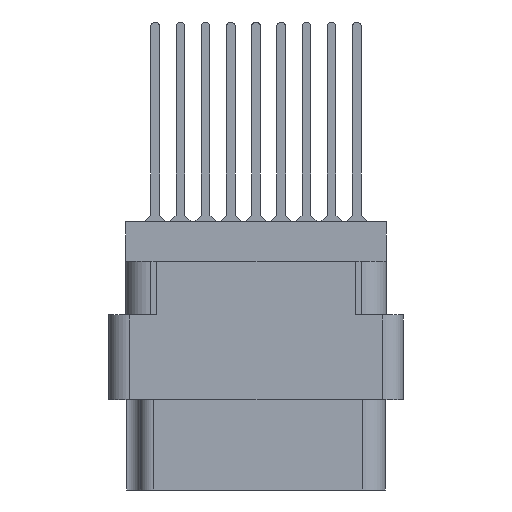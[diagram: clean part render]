
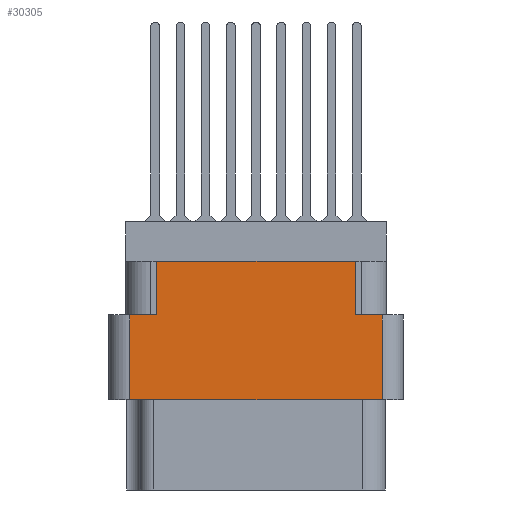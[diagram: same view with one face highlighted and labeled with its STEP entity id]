
A CAD part, left-side view. The second image highlights one B-rep face of the part: STEP entity #30305.
In plain terms, the highlighted planar face has unit normal (-1, 0, 0).
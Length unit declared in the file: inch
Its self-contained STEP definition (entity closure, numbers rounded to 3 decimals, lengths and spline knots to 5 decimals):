
#547 = CARTESIAN_POINT ( 'NONE',  ( -1.296, -0.296, -0.117 ) ) ;
#1099 = CARTESIAN_POINT ( 'NONE',  ( -1.296, -0.438, -0.798 ) ) ;
#1551 = LINE ( 'NONE', #26097, #23637 ) ;
#1974 = DIRECTION ( 'NONE',  ( 0., -1., 0. ) ) ;
#1977 = VECTOR ( 'NONE', #12598, 39.37008 ) ;
#2829 = FACE_OUTER_BOUND ( 'NONE', #41896, .T. ) ;
#2969 = EDGE_CURVE ( 'NONE', #28040, #22588, #7296, .T. ) ;
#3328 = CARTESIAN_POINT ( 'NONE',  ( -1.296, 0.376, -0.529 ) ) ;
#3400 = DIRECTION ( 'NONE',  ( 0., 0., 1. ) ) ;
#4761 = CARTESIAN_POINT ( 'NONE',  ( -1.296, -0.376, -0.277 ) ) ;
#4982 = DIRECTION ( 'NONE',  ( 0., -1., 0. ) ) ;
#5365 = CARTESIAN_POINT ( 'NONE',  ( -1.296, -0.376, -0.529 ) ) ;
#5426 = CARTESIAN_POINT ( 'NONE',  ( -1.296, 0., -0.277 ) ) ;
#5723 = CARTESIAN_POINT ( 'NONE',  ( -1.296, -0.376, -0.798 ) ) ;
#6245 = CARTESIAN_POINT ( 'NONE',  ( -1.296, 0., -0.277 ) ) ;
#6827 = ORIENTED_EDGE ( 'NONE', *, *, #17819, .F. ) ;
#7296 = LINE ( 'NONE', #6245, #36928 ) ;
#8080 = ORIENTED_EDGE ( 'NONE', *, *, #15998, .F. ) ;
#8143 = LINE ( 'NONE', #5723, #31485 ) ;
#8845 = EDGE_CURVE ( 'NONE', #33349, #35713, #40647, .T. ) ;
#8875 = LINE ( 'NONE', #35286, #36778 ) ;
#9714 = CARTESIAN_POINT ( 'NONE',  ( -1.296, 0.296, -0.277 ) ) ;
#10306 = ORIENTED_EDGE ( 'NONE', *, *, #16696, .F. ) ;
#10911 = ORIENTED_EDGE ( 'NONE', *, *, #2969, .F. ) ;
#11668 = LINE ( 'NONE', #5426, #1977 ) ;
#11887 = AXIS2_PLACEMENT_3D ( 'NONE', #1099, #27017, #30865 ) ;
#12366 = VERTEX_POINT ( 'NONE', #5365 ) ;
#12598 = DIRECTION ( 'NONE',  ( 0., -1., 0. ) ) ;
#13637 = CARTESIAN_POINT ( 'NONE',  ( -1.296, 0.296, -0.117 ) ) ;
#14191 = LINE ( 'NONE', #25764, #42053 ) ;
#15232 = VERTEX_POINT ( 'NONE', #3328 ) ;
#15998 = EDGE_CURVE ( 'NONE', #46280, #35713, #31086, .T. ) ;
#16094 = ORIENTED_EDGE ( 'NONE', *, *, #34705, .T. ) ;
#16419 = VERTEX_POINT ( 'NONE', #4761 ) ;
#16696 = EDGE_CURVE ( 'NONE', #22588, #46280, #8875, .T. ) ;
#17819 = EDGE_CURVE ( 'NONE', #33349, #16419, #11668, .T. ) ;
#18275 = DIRECTION ( 'NONE',  ( 0., 1., 0. ) ) ;
#18349 = CARTESIAN_POINT ( 'NONE',  ( -1.296, 0.438, -0.117 ) ) ;
#22588 = VERTEX_POINT ( 'NONE', #9714 ) ;
#23216 = PLANE ( 'NONE',  #11887 ) ;
#23637 = VECTOR ( 'NONE', #26418, 39.37008 ) ;
#24332 = DIRECTION ( 'NONE',  ( 0., 0., 1. ) ) ;
#25764 = CARTESIAN_POINT ( 'NONE',  ( -1.296, 0., -0.529 ) ) ;
#26097 = CARTESIAN_POINT ( 'NONE',  ( -1.296, 0.376, -0.798 ) ) ;
#26418 = DIRECTION ( 'NONE',  ( 0., 0., -1. ) ) ;
#27017 = DIRECTION ( 'NONE',  ( -1., 0., 0. ) ) ;
#28040 = VERTEX_POINT ( 'NONE', #42816 ) ;
#30305 = ADVANCED_FACE ( 'NONE', ( #2829 ), #23216, .T. ) ;
#30865 = DIRECTION ( 'NONE',  ( 0., 0., 1. ) ) ;
#31086 = LINE ( 'NONE', #18349, #40736 ) ;
#31370 = ORIENTED_EDGE ( 'NONE', *, *, #43304, .F. ) ;
#31485 = VECTOR ( 'NONE', #24332, 39.37008 ) ;
#32845 = CARTESIAN_POINT ( 'NONE',  ( -1.296, -0.296, -0.277 ) ) ;
#33349 = VERTEX_POINT ( 'NONE', #46188 ) ;
#34429 = ORIENTED_EDGE ( 'NONE', *, *, #36797, .T. ) ;
#34705 = EDGE_CURVE ( 'NONE', #12366, #16419, #8143, .T. ) ;
#34960 = ORIENTED_EDGE ( 'NONE', *, *, #8845, .T. ) ;
#35286 = CARTESIAN_POINT ( 'NONE',  ( -1.296, 0.296, -0.277 ) ) ;
#35713 = VERTEX_POINT ( 'NONE', #547 ) ;
#36778 = VECTOR ( 'NONE', #45808, 39.37008 ) ;
#36797 = EDGE_CURVE ( 'NONE', #28040, #15232, #1551, .T. ) ;
#36928 = VECTOR ( 'NONE', #1974, 39.37008 ) ;
#40647 = LINE ( 'NONE', #32845, #41247 ) ;
#40736 = VECTOR ( 'NONE', #4982, 39.37008 ) ;
#41247 = VECTOR ( 'NONE', #3400, 39.37008 ) ;
#41896 = EDGE_LOOP ( 'NONE', ( #10911, #34429, #31370, #16094, #6827, #34960, #8080, #10306 ) ) ;
#42053 = VECTOR ( 'NONE', #18275, 39.37008 ) ;
#42816 = CARTESIAN_POINT ( 'NONE',  ( -1.296, 0.376, -0.277 ) ) ;
#43304 = EDGE_CURVE ( 'NONE', #12366, #15232, #14191, .T. ) ;
#45808 = DIRECTION ( 'NONE',  ( 0., 0., 1. ) ) ;
#46188 = CARTESIAN_POINT ( 'NONE',  ( -1.296, -0.296, -0.277 ) ) ;
#46280 = VERTEX_POINT ( 'NONE', #13637 ) ;
